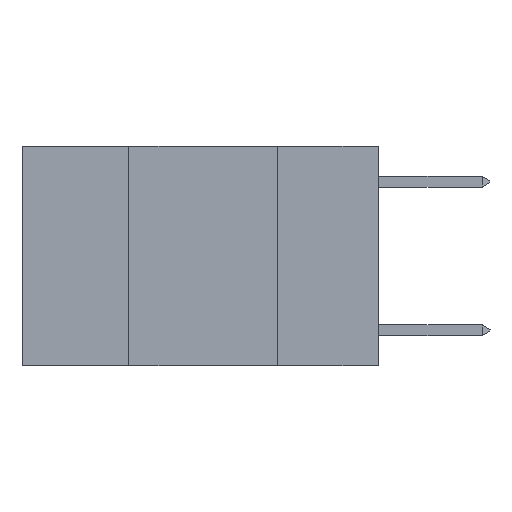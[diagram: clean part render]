
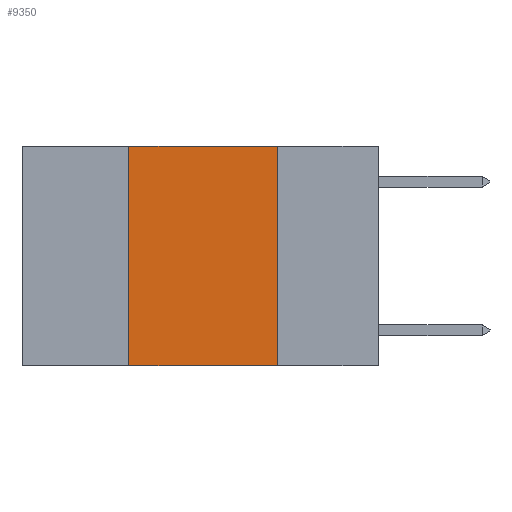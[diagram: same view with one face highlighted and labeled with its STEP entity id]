
A CAD part, left-side view. The second image highlights one B-rep face of the part: STEP entity #9350.
In plain terms, the highlighted planar face has unit normal (-1, 0, 0).
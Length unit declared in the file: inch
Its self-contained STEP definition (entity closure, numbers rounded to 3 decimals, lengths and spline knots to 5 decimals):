
#400 = DIRECTION ( 'NONE',  ( 0., 0., -1. ) ) ;
#703 = ORIENTED_EDGE ( 'NONE', *, *, #12246, .F. ) ;
#826 = LINE ( 'NONE', #3599, #3488 ) ;
#1083 = ORIENTED_EDGE ( 'NONE', *, *, #5987, .F. ) ;
#1313 = FACE_OUTER_BOUND ( 'NONE', #13641, .T. ) ;
#1564 = EDGE_CURVE ( 'NONE', #13065, #8009, #826, .T. ) ;
#1803 = ORIENTED_EDGE ( 'NONE', *, *, #1564, .F. ) ;
#1890 = VERTEX_POINT ( 'NONE', #3034 ) ;
#2303 = VECTOR ( 'NONE', #3660, 39.37008 ) ;
#3034 = CARTESIAN_POINT ( 'NONE',  ( 0., 0.17, -0.37 ) ) ;
#3488 = VECTOR ( 'NONE', #8071, 39.37008 ) ;
#3599 = CARTESIAN_POINT ( 'NONE',  ( 0., 0.42, 0. ) ) ;
#3660 = DIRECTION ( 'NONE',  ( 0., -1., 0. ) ) ;
#4052 = DIRECTION ( 'NONE',  ( 0., -1., 0. ) ) ;
#4536 = AXIS2_PLACEMENT_3D ( 'NONE', #13685, #7197, #400 ) ;
#5517 = ORIENTED_EDGE ( 'NONE', *, *, #13011, .T. ) ;
#5987 = EDGE_CURVE ( 'NONE', #8009, #12054, #9855, .T. ) ;
#6069 = PLANE ( 'NONE',  #4536 ) ;
#6917 = VECTOR ( 'NONE', #4052, 39.37008 ) ;
#7197 = DIRECTION ( 'NONE',  ( 1., 0., 0. ) ) ;
#8009 = VERTEX_POINT ( 'NONE', #9252 ) ;
#8071 = DIRECTION ( 'NONE',  ( 0., 0., 1. ) ) ;
#8228 = CARTESIAN_POINT ( 'NONE',  ( 0., 0.42, -0.37 ) ) ;
#8429 = DIRECTION ( 'NONE',  ( 0., 0., -1. ) ) ;
#8651 = LINE ( 'NONE', #13518, #2303 ) ;
#9252 = CARTESIAN_POINT ( 'NONE',  ( 0., 0.42, 0. ) ) ;
#9350 = ADVANCED_FACE ( 'NONE', ( #1313 ), #6069, .F. ) ;
#9690 = VECTOR ( 'NONE', #8429, 39.37008 ) ;
#9855 = LINE ( 'NONE', #10698, #6917 ) ;
#10698 = CARTESIAN_POINT ( 'NONE',  ( 0., 0.6, 0. ) ) ;
#11664 = CARTESIAN_POINT ( 'NONE',  ( 0., 0.17, 0. ) ) ;
#12054 = VERTEX_POINT ( 'NONE', #13522 ) ;
#12246 = EDGE_CURVE ( 'NONE', #12054, #1890, #12540, .T. ) ;
#12540 = LINE ( 'NONE', #11664, #9690 ) ;
#13011 = EDGE_CURVE ( 'NONE', #13065, #1890, #8651, .T. ) ;
#13065 = VERTEX_POINT ( 'NONE', #8228 ) ;
#13518 = CARTESIAN_POINT ( 'NONE',  ( 0., 0.6, -0.37 ) ) ;
#13522 = CARTESIAN_POINT ( 'NONE',  ( 0., 0.17, 0. ) ) ;
#13641 = EDGE_LOOP ( 'NONE', ( #703, #1083, #1803, #5517 ) ) ;
#13685 = CARTESIAN_POINT ( 'NONE',  ( 0., 0.6, 0. ) ) ;
